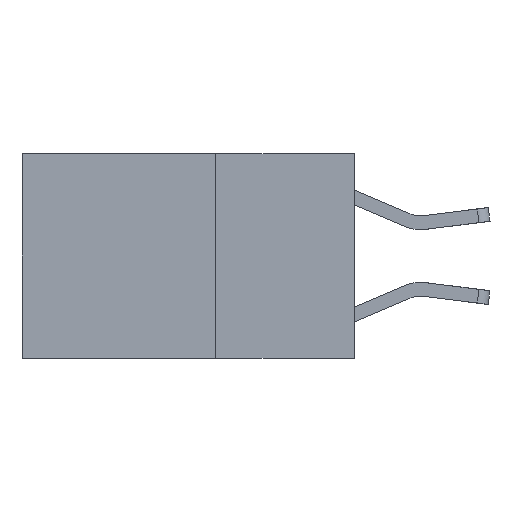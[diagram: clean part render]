
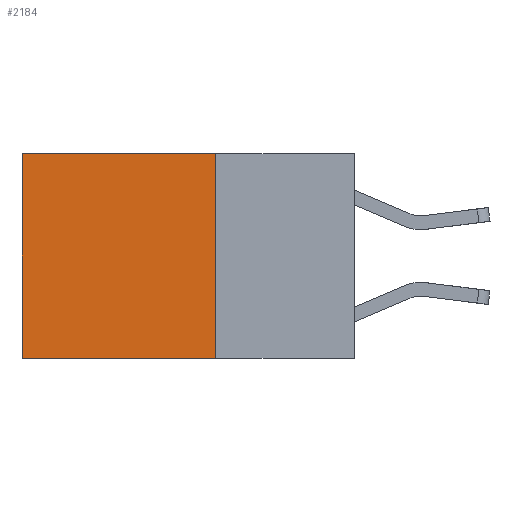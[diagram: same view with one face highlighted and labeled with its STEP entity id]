
A CAD part, left-side view. The second image highlights one B-rep face of the part: STEP entity #2184.
In plain terms, the highlighted planar face has unit normal (-1, 0, 0).
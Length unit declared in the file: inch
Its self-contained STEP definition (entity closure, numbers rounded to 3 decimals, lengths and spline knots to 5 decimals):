
#297 = VERTEX_POINT ( 'NONE', #3989 ) ;
#439 = VERTEX_POINT ( 'NONE', #1615 ) ;
#550 = PLANE ( 'NONE',  #2816 ) ;
#610 = VECTOR ( 'NONE', #4660, 39.37008 ) ;
#876 = LINE ( 'NONE', #7656, #7192 ) ;
#1032 = DIRECTION ( 'NONE',  ( 0., 0., -1. ) ) ;
#1615 = CARTESIAN_POINT ( 'NONE',  ( 0.2625, 0.6, 0. ) ) ;
#1872 = VERTEX_POINT ( 'NONE', #8276 ) ;
#2184 = ADVANCED_FACE ( 'NONE', ( #5021 ), #550, .F. ) ;
#2816 = AXIS2_PLACEMENT_3D ( 'NONE', #7158, #3172, #8777 ) ;
#3050 = ORIENTED_EDGE ( 'NONE', *, *, #9080, .F. ) ;
#3172 = DIRECTION ( 'NONE',  ( 1., 0., 0. ) ) ;
#3989 = CARTESIAN_POINT ( 'NONE',  ( 0.2625, 0.25, -0.37 ) ) ;
#4660 = DIRECTION ( 'NONE',  ( 0., 1., 0. ) ) ;
#4665 = CARTESIAN_POINT ( 'NONE',  ( 0.2625, 0.25, 0. ) ) ;
#4717 = LINE ( 'NONE', #4665, #8691 ) ;
#4857 = LINE ( 'NONE', #9423, #610 ) ;
#4893 = CARTESIAN_POINT ( 'NONE',  ( 0.2625, 0.6, -0.37 ) ) ;
#5021 = FACE_OUTER_BOUND ( 'NONE', #9570, .T. ) ;
#5291 = DIRECTION ( 'NONE',  ( 0., 0., -1. ) ) ;
#5601 = VECTOR ( 'NONE', #1032, 39.37008 ) ;
#5880 = VERTEX_POINT ( 'NONE', #4893 ) ;
#7158 = CARTESIAN_POINT ( 'NONE',  ( 0.2625, 0.25, 0. ) ) ;
#7192 = VECTOR ( 'NONE', #5291, 39.37008 ) ;
#7656 = CARTESIAN_POINT ( 'NONE',  ( 0.2625, 0.6, 0. ) ) ;
#7662 = ORIENTED_EDGE ( 'NONE', *, *, #10526, .T. ) ;
#7696 = LINE ( 'NONE', #8368, #5601 ) ;
#8251 = ORIENTED_EDGE ( 'NONE', *, *, #8736, .F. ) ;
#8276 = CARTESIAN_POINT ( 'NONE',  ( 0.2625, 0.25, 0. ) ) ;
#8368 = CARTESIAN_POINT ( 'NONE',  ( 0.2625, 0.25, 0. ) ) ;
#8691 = VECTOR ( 'NONE', #9461, 39.37008 ) ;
#8736 = EDGE_CURVE ( 'NONE', #297, #5880, #4857, .T. ) ;
#8777 = DIRECTION ( 'NONE',  ( 0., 0., -1. ) ) ;
#9080 = EDGE_CURVE ( 'NONE', #1872, #297, #7696, .T. ) ;
#9137 = EDGE_CURVE ( 'NONE', #439, #5880, #876, .T. ) ;
#9270 = ORIENTED_EDGE ( 'NONE', *, *, #9137, .T. ) ;
#9423 = CARTESIAN_POINT ( 'NONE',  ( 0.2625, 0.25, -0.37 ) ) ;
#9461 = DIRECTION ( 'NONE',  ( 0., 1., 0. ) ) ;
#9570 = EDGE_LOOP ( 'NONE', ( #9270, #8251, #3050, #7662 ) ) ;
#10526 = EDGE_CURVE ( 'NONE', #1872, #439, #4717, .T. ) ;
